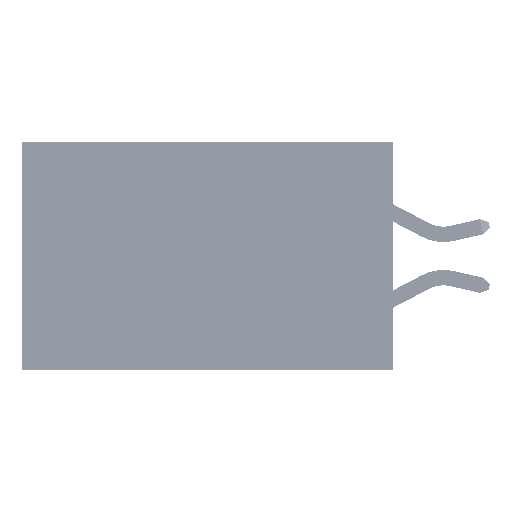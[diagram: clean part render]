
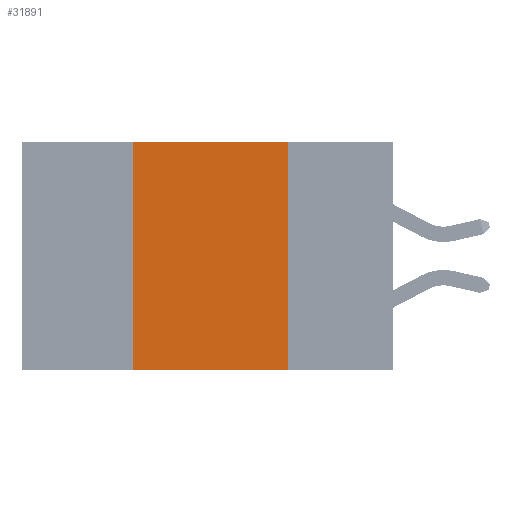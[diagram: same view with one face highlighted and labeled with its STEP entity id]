
A CAD part, left-side view. The second image highlights one B-rep face of the part: STEP entity #31891.
In plain terms, the highlighted planar face has unit normal (-1, 0, 0).
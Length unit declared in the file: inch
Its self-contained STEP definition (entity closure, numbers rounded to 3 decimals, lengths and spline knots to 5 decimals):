
#469 = AXIS2_PLACEMENT_3D ( 'NONE', #46645, #20961, #1152 ) ;
#1152 = DIRECTION ( 'NONE',  ( 0., 0., -1. ) ) ;
#1313 = VECTOR ( 'NONE', #42016, 39.37008 ) ;
#1993 = DIRECTION ( 'NONE',  ( 0., -1., 0. ) ) ;
#2405 = LINE ( 'NONE', #16860, #21398 ) ;
#3770 = VERTEX_POINT ( 'NONE', #43588 ) ;
#5064 = DIRECTION ( 'NONE',  ( 0., 0., -1. ) ) ;
#5853 = ORIENTED_EDGE ( 'NONE', *, *, #38142, .F. ) ;
#6700 = VERTEX_POINT ( 'NONE', #14908 ) ;
#14079 = VECTOR ( 'NONE', #28099, 39.37008 ) ;
#14908 = CARTESIAN_POINT ( 'NONE',  ( 0., 0.17, -0.37 ) ) ;
#16007 = PLANE ( 'NONE',  #469 ) ;
#16218 = CARTESIAN_POINT ( 'NONE',  ( 0., 0.17, 0. ) ) ;
#16860 = CARTESIAN_POINT ( 'NONE',  ( 0., 0.6, -0.37 ) ) ;
#20757 = VERTEX_POINT ( 'NONE', #36989 ) ;
#20919 = LINE ( 'NONE', #34932, #1313 ) ;
#20961 = DIRECTION ( 'NONE',  ( 1., 0., 0. ) ) ;
#21398 = VECTOR ( 'NONE', #1993, 39.37008 ) ;
#22482 = LINE ( 'NONE', #41316, #38590 ) ;
#22950 = EDGE_CURVE ( 'NONE', #20757, #3770, #33613, .T. ) ;
#27232 = ORIENTED_EDGE ( 'NONE', *, *, #47100, .F. ) ;
#28099 = DIRECTION ( 'NONE',  ( 0., 0., 1. ) ) ;
#30174 = VERTEX_POINT ( 'NONE', #16218 ) ;
#31416 = EDGE_CURVE ( 'NONE', #20757, #6700, #2405, .T. ) ;
#31891 = ADVANCED_FACE ( 'NONE', ( #44466 ), #16007, .F. ) ;
#32463 = ORIENTED_EDGE ( 'NONE', *, *, #22950, .F. ) ;
#33613 = LINE ( 'NONE', #35846, #14079 ) ;
#33876 = ORIENTED_EDGE ( 'NONE', *, *, #31416, .T. ) ;
#34932 = CARTESIAN_POINT ( 'NONE',  ( 0., 0.6, 0. ) ) ;
#35846 = CARTESIAN_POINT ( 'NONE',  ( 0., 0.42, 0. ) ) ;
#36989 = CARTESIAN_POINT ( 'NONE',  ( 0., 0.42, -0.37 ) ) ;
#38142 = EDGE_CURVE ( 'NONE', #30174, #6700, #22482, .T. ) ;
#38590 = VECTOR ( 'NONE', #5064, 39.37008 ) ;
#40580 = EDGE_LOOP ( 'NONE', ( #5853, #27232, #32463, #33876 ) ) ;
#41316 = CARTESIAN_POINT ( 'NONE',  ( 0., 0.17, 0. ) ) ;
#42016 = DIRECTION ( 'NONE',  ( 0., -1., 0. ) ) ;
#43588 = CARTESIAN_POINT ( 'NONE',  ( 0., 0.42, 0. ) ) ;
#44466 = FACE_OUTER_BOUND ( 'NONE', #40580, .T. ) ;
#46645 = CARTESIAN_POINT ( 'NONE',  ( 0., 0.6, 0. ) ) ;
#47100 = EDGE_CURVE ( 'NONE', #3770, #30174, #20919, .T. ) ;
